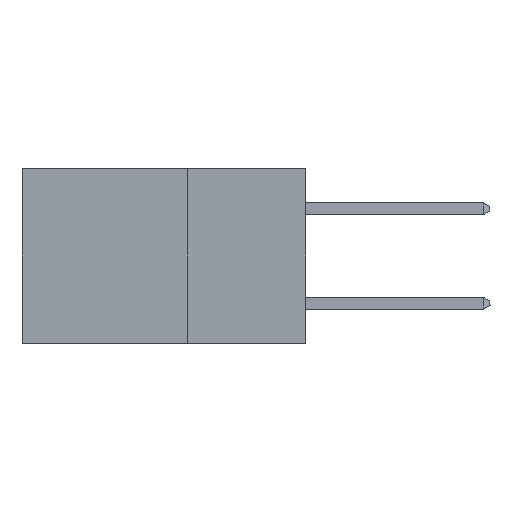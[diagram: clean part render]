
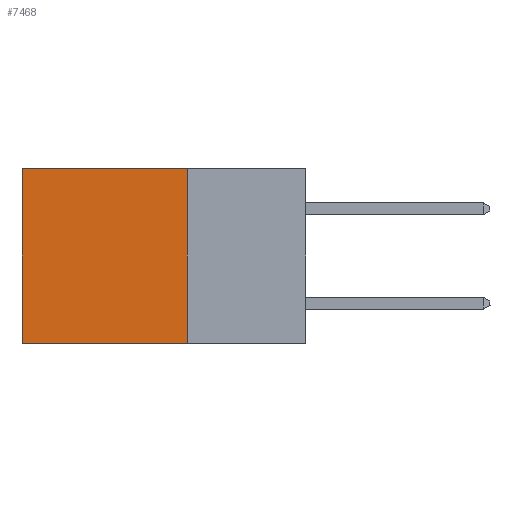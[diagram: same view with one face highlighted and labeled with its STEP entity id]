
A CAD part, left-side view. The second image highlights one B-rep face of the part: STEP entity #7468.
In plain terms, the highlighted planar face has unit normal (-1, 0, 0).
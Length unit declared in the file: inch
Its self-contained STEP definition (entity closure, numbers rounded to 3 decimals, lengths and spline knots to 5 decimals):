
#241 = CARTESIAN_POINT ( 'NONE',  ( 0.298, 0.25, -0.37 ) ) ;
#1638 = CARTESIAN_POINT ( 'NONE',  ( 0.298, 0.25, 0. ) ) ;
#2561 = EDGE_CURVE ( 'NONE', #27127, #5266, #10534, .T. ) ;
#2868 = ORIENTED_EDGE ( 'NONE', *, *, #27075, .F. ) ;
#4563 = EDGE_CURVE ( 'NONE', #15185, #28764, #11356, .T. ) ;
#5266 = VERTEX_POINT ( 'NONE', #20108 ) ;
#5713 = ORIENTED_EDGE ( 'NONE', *, *, #21328, .T. ) ;
#6331 = DIRECTION ( 'NONE',  ( 0., 0., -1. ) ) ;
#7468 = ADVANCED_FACE ( 'NONE', ( #13573 ), #31259, .F. ) ;
#8502 = DIRECTION ( 'NONE',  ( 0., 0., -1. ) ) ;
#9991 = EDGE_LOOP ( 'NONE', ( #5713, #31569, #2868, #17888 ) ) ;
#10534 = LINE ( 'NONE', #22034, #29336 ) ;
#11356 = LINE ( 'NONE', #20299, #23728 ) ;
#13426 = VECTOR ( 'NONE', #8502, 39.37008 ) ;
#13573 = FACE_OUTER_BOUND ( 'NONE', #9991, .T. ) ;
#13919 = CARTESIAN_POINT ( 'NONE',  ( 0.298, 0.25, 0. ) ) ;
#14679 = LINE ( 'NONE', #13919, #26151 ) ;
#15185 = VERTEX_POINT ( 'NONE', #241 ) ;
#15680 = CARTESIAN_POINT ( 'NONE',  ( 0.298, 0.6, -0.37 ) ) ;
#16144 = CARTESIAN_POINT ( 'NONE',  ( 0.298, 0.25, 0. ) ) ;
#17888 = ORIENTED_EDGE ( 'NONE', *, *, #2561, .T. ) ;
#20108 = CARTESIAN_POINT ( 'NONE',  ( 0.298, 0.6, 0. ) ) ;
#20299 = CARTESIAN_POINT ( 'NONE',  ( 0.298, 0.25, -0.37 ) ) ;
#20566 = DIRECTION ( 'NONE',  ( 0., 1., 0. ) ) ;
#21328 = EDGE_CURVE ( 'NONE', #5266, #28764, #25673, .T. ) ;
#22034 = CARTESIAN_POINT ( 'NONE',  ( 0.298, 0.25, 0. ) ) ;
#23728 = VECTOR ( 'NONE', #31310, 39.37008 ) ;
#25673 = LINE ( 'NONE', #28132, #13426 ) ;
#26151 = VECTOR ( 'NONE', #6331, 39.37008 ) ;
#27075 = EDGE_CURVE ( 'NONE', #27127, #15185, #14679, .T. ) ;
#27127 = VERTEX_POINT ( 'NONE', #1638 ) ;
#28132 = CARTESIAN_POINT ( 'NONE',  ( 0.298, 0.6, 0. ) ) ;
#28764 = VERTEX_POINT ( 'NONE', #15680 ) ;
#28904 = DIRECTION ( 'NONE',  ( 0., 0., -1. ) ) ;
#29026 = AXIS2_PLACEMENT_3D ( 'NONE', #16144, #31162, #28904 ) ;
#29336 = VECTOR ( 'NONE', #20566, 39.37008 ) ;
#31162 = DIRECTION ( 'NONE',  ( 1., 0., 0. ) ) ;
#31259 = PLANE ( 'NONE',  #29026 ) ;
#31310 = DIRECTION ( 'NONE',  ( 0., 1., 0. ) ) ;
#31569 = ORIENTED_EDGE ( 'NONE', *, *, #4563, .F. ) ;
